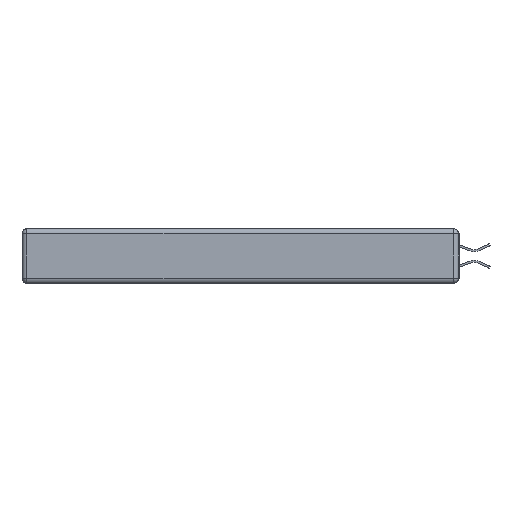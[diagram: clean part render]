
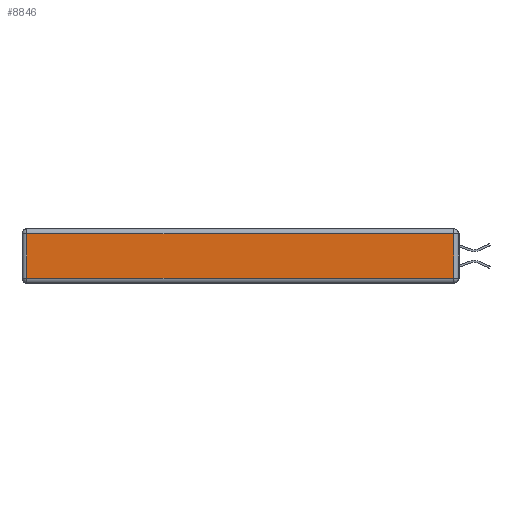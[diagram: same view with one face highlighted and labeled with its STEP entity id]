
A CAD part, left-side view. The second image highlights one B-rep face of the part: STEP entity #8846.
In plain terms, the highlighted planar face has unit normal (-1, 0, 0).
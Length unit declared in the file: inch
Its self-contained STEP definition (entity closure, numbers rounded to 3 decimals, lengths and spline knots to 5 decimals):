
#447 = VERTEX_POINT ( 'NONE', #15587 ) ;
#763 = LINE ( 'NONE', #5174, #18498 ) ;
#1017 = DIRECTION ( 'NONE',  ( -1., 0., 0. ) ) ;
#2130 = EDGE_CURVE ( 'NONE', #15352, #13952, #10065, .T. ) ;
#2426 = DIRECTION ( 'NONE',  ( 0., 1., 0. ) ) ;
#3047 = CARTESIAN_POINT ( 'NONE',  ( 0., 0., -0.343 ) ) ;
#5107 = DIRECTION ( 'NONE',  ( 0., 0., 1. ) ) ;
#5174 = CARTESIAN_POINT ( 'NONE',  ( 0., 0., -0.313 ) ) ;
#7588 = DIRECTION ( 'NONE',  ( 0., 0., 1. ) ) ;
#7909 = VECTOR ( 'NONE', #2426, 39.37008 ) ;
#8846 = ADVANCED_FACE ( 'NONE', ( #13974 ), #12082, .T. ) ;
#9162 = DIRECTION ( 'NONE',  ( 0., -1., 0. ) ) ;
#9475 = CARTESIAN_POINT ( 'NONE',  ( 0., 2.72, -0.343 ) ) ;
#10065 = LINE ( 'NONE', #26785, #26818 ) ;
#10311 = LINE ( 'NONE', #19780, #7909 ) ;
#11201 = CARTESIAN_POINT ( 'NONE',  ( 0., 0.03, -0.313 ) ) ;
#12082 = PLANE ( 'NONE',  #14003 ) ;
#12563 = ORIENTED_EDGE ( 'NONE', *, *, #2130, .T. ) ;
#12882 = ORIENTED_EDGE ( 'NONE', *, *, #23887, .T. ) ;
#13952 = VERTEX_POINT ( 'NONE', #17018 ) ;
#13974 = FACE_OUTER_BOUND ( 'NONE', #27935, .T. ) ;
#14003 = AXIS2_PLACEMENT_3D ( 'NONE', #3047, #1017, #7588 ) ;
#14280 = ORIENTED_EDGE ( 'NONE', *, *, #21461, .T. ) ;
#15352 = VERTEX_POINT ( 'NONE', #11201 ) ;
#15587 = CARTESIAN_POINT ( 'NONE',  ( 0., 2.72, -0.313 ) ) ;
#17018 = CARTESIAN_POINT ( 'NONE',  ( 0., 0.03, -0.03 ) ) ;
#17590 = ORIENTED_EDGE ( 'NONE', *, *, #28254, .T. ) ;
#18498 = VECTOR ( 'NONE', #9162, 39.37008 ) ;
#18577 = VERTEX_POINT ( 'NONE', #18615 ) ;
#18615 = CARTESIAN_POINT ( 'NONE',  ( 0., 2.72, -0.03 ) ) ;
#19780 = CARTESIAN_POINT ( 'NONE',  ( 0., 2.75, -0.03 ) ) ;
#21461 = EDGE_CURVE ( 'NONE', #18577, #447, #22388, .T. ) ;
#22388 = LINE ( 'NONE', #9475, #23074 ) ;
#23074 = VECTOR ( 'NONE', #24743, 39.37008 ) ;
#23887 = EDGE_CURVE ( 'NONE', #13952, #18577, #10311, .T. ) ;
#24743 = DIRECTION ( 'NONE',  ( 0., 0., -1. ) ) ;
#26785 = CARTESIAN_POINT ( 'NONE',  ( 0., 0.03, -0.343 ) ) ;
#26818 = VECTOR ( 'NONE', #5107, 39.37008 ) ;
#27935 = EDGE_LOOP ( 'NONE', ( #17590, #12563, #12882, #14280 ) ) ;
#28254 = EDGE_CURVE ( 'NONE', #447, #15352, #763, .T. ) ;
